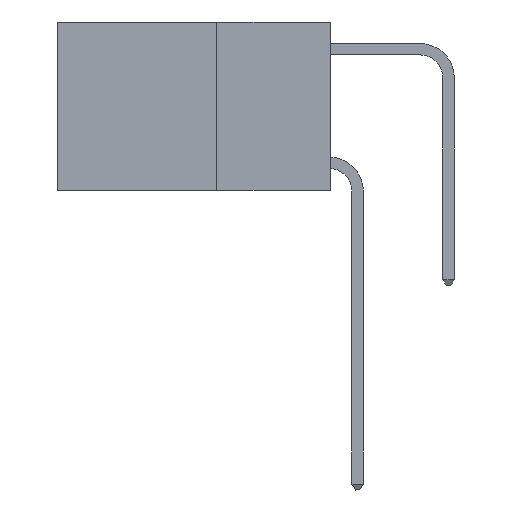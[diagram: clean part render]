
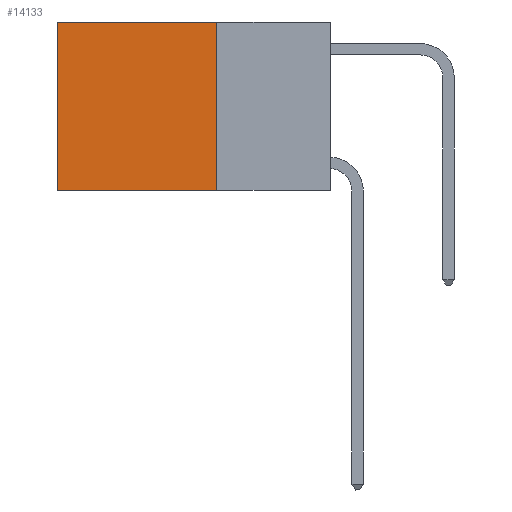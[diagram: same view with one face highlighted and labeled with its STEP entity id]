
A CAD part, left-side view. The second image highlights one B-rep face of the part: STEP entity #14133.
In plain terms, the highlighted planar face has unit normal (-1, 0, 0).
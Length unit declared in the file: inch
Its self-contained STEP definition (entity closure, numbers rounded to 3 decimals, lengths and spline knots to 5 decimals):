
#1009 = DIRECTION ( 'NONE',  ( 0., 1., 0. ) ) ;
#2710 = EDGE_CURVE ( 'NONE', #15338, #10422, #13432, .T. ) ;
#4577 = VECTOR ( 'NONE', #1009, 39.37008 ) ;
#5456 = CARTESIAN_POINT ( 'NONE',  ( 0.2625, 0.6, 0. ) ) ;
#6868 = CARTESIAN_POINT ( 'NONE',  ( 0.2625, 0.6, 0. ) ) ;
#8295 = CARTESIAN_POINT ( 'NONE',  ( 0.2625, 0.25, -0.37 ) ) ;
#8356 = PLANE ( 'NONE',  #24244 ) ;
#8369 = VECTOR ( 'NONE', #24436, 39.37008 ) ;
#9982 = CARTESIAN_POINT ( 'NONE',  ( 0.2625, 0.25, -0.37 ) ) ;
#10422 = VERTEX_POINT ( 'NONE', #5456 ) ;
#11157 = VERTEX_POINT ( 'NONE', #9982 ) ;
#11842 = ORIENTED_EDGE ( 'NONE', *, *, #18966, .T. ) ;
#12169 = VECTOR ( 'NONE', #14801, 39.37008 ) ;
#13432 = LINE ( 'NONE', #23734, #4577 ) ;
#13483 = DIRECTION ( 'NONE',  ( 1., 0., 0. ) ) ;
#14133 = ADVANCED_FACE ( 'NONE', ( #20950 ), #8356, .F. ) ;
#14801 = DIRECTION ( 'NONE',  ( 0., 0., -1. ) ) ;
#15338 = VERTEX_POINT ( 'NONE', #22442 ) ;
#15964 = CARTESIAN_POINT ( 'NONE',  ( 0.2625, 0.25, 0. ) ) ;
#16095 = ORIENTED_EDGE ( 'NONE', *, *, #30267, .F. ) ;
#16356 = ORIENTED_EDGE ( 'NONE', *, *, #27265, .F. ) ;
#17976 = DIRECTION ( 'NONE',  ( 0., 0., -1. ) ) ;
#18017 = EDGE_LOOP ( 'NONE', ( #11842, #16356, #16095, #32109 ) ) ;
#18966 = EDGE_CURVE ( 'NONE', #10422, #28123, #26794, .T. ) ;
#20950 = FACE_OUTER_BOUND ( 'NONE', #18017, .T. ) ;
#21836 = CARTESIAN_POINT ( 'NONE',  ( 0.2625, 0.6, -0.37 ) ) ;
#22442 = CARTESIAN_POINT ( 'NONE',  ( 0.2625, 0.25, 0. ) ) ;
#23239 = LINE ( 'NONE', #8295, #23601 ) ;
#23601 = VECTOR ( 'NONE', #25579, 39.37008 ) ;
#23734 = CARTESIAN_POINT ( 'NONE',  ( 0.2625, 0.25, 0. ) ) ;
#24244 = AXIS2_PLACEMENT_3D ( 'NONE', #15964, #13483, #17976 ) ;
#24436 = DIRECTION ( 'NONE',  ( 0., 0., -1. ) ) ;
#25579 = DIRECTION ( 'NONE',  ( 0., 1., 0. ) ) ;
#26768 = CARTESIAN_POINT ( 'NONE',  ( 0.2625, 0.25, 0. ) ) ;
#26794 = LINE ( 'NONE', #6868, #12169 ) ;
#27265 = EDGE_CURVE ( 'NONE', #11157, #28123, #23239, .T. ) ;
#28123 = VERTEX_POINT ( 'NONE', #21836 ) ;
#29886 = LINE ( 'NONE', #26768, #8369 ) ;
#30267 = EDGE_CURVE ( 'NONE', #15338, #11157, #29886, .T. ) ;
#32109 = ORIENTED_EDGE ( 'NONE', *, *, #2710, .T. ) ;
